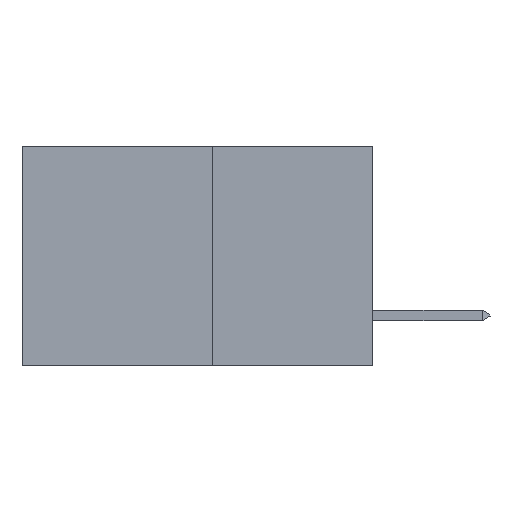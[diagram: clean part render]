
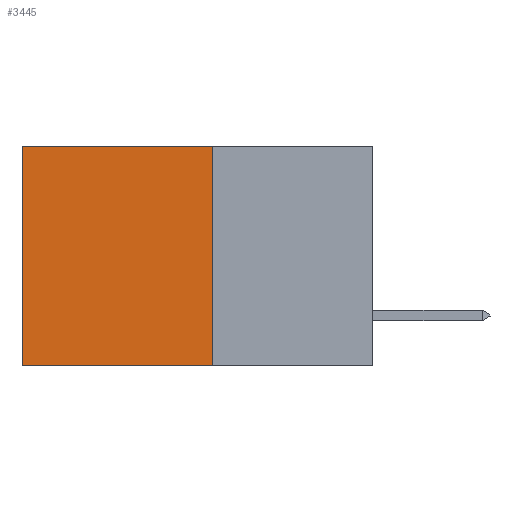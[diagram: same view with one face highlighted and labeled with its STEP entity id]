
A CAD part, left-side view. The second image highlights one B-rep face of the part: STEP entity #3445.
In plain terms, the highlighted planar face has unit normal (-1, 0, 0).
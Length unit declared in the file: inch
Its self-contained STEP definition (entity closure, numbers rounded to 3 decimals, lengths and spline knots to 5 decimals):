
#724 = ORIENTED_EDGE ( 'NONE', *, *, #5839, .F. ) ;
#1771 = VERTEX_POINT ( 'NONE', #5161 ) ;
#1816 = DIRECTION ( 'NONE',  ( 0., 0., -1. ) ) ;
#1899 = DIRECTION ( 'NONE',  ( 1., 0., 0. ) ) ;
#2190 = DIRECTION ( 'NONE',  ( 0., 1., 0. ) ) ;
#2387 = LINE ( 'NONE', #5983, #12265 ) ;
#2451 = PLANE ( 'NONE',  #14205 ) ;
#2814 = VECTOR ( 'NONE', #15606, 39.37008 ) ;
#2825 = CARTESIAN_POINT ( 'NONE',  ( 0.277, 0.27, -0.37 ) ) ;
#2922 = CARTESIAN_POINT ( 'NONE',  ( 0.277, 0.27, -0.37 ) ) ;
#3444 = EDGE_CURVE ( 'NONE', #1771, #4629, #15826, .T. ) ;
#3445 = ADVANCED_FACE ( 'NONE', ( #6402 ), #2451, .F. ) ;
#4629 = VERTEX_POINT ( 'NONE', #6544 ) ;
#5161 = CARTESIAN_POINT ( 'NONE',  ( 0.277, 0.27, -0.37 ) ) ;
#5839 = EDGE_CURVE ( 'NONE', #7050, #1771, #9433, .T. ) ;
#5983 = CARTESIAN_POINT ( 'NONE',  ( 0.277, 0.59, -0.37 ) ) ;
#6402 = FACE_OUTER_BOUND ( 'NONE', #15856, .T. ) ;
#6544 = CARTESIAN_POINT ( 'NONE',  ( 0.277, 0.59, -0.37 ) ) ;
#7050 = VERTEX_POINT ( 'NONE', #11337 ) ;
#7875 = VECTOR ( 'NONE', #11396, 39.37008 ) ;
#8386 = VERTEX_POINT ( 'NONE', #10908 ) ;
#9433 = LINE ( 'NONE', #15639, #2814 ) ;
#10185 = CARTESIAN_POINT ( 'NONE',  ( 0.277, 0.27, 0. ) ) ;
#10723 = ORIENTED_EDGE ( 'NONE', *, *, #13278, .T. ) ;
#10900 = DIRECTION ( 'NONE',  ( 0., 0., -1. ) ) ;
#10908 = CARTESIAN_POINT ( 'NONE',  ( 0.277, 0.59, 0. ) ) ;
#11141 = LINE ( 'NONE', #10185, #7875 ) ;
#11337 = CARTESIAN_POINT ( 'NONE',  ( 0.277, 0.27, 0. ) ) ;
#11396 = DIRECTION ( 'NONE',  ( 0., 1., 0. ) ) ;
#11452 = ORIENTED_EDGE ( 'NONE', *, *, #14411, .T. ) ;
#11821 = ORIENTED_EDGE ( 'NONE', *, *, #3444, .F. ) ;
#12265 = VECTOR ( 'NONE', #10900, 39.37008 ) ;
#12534 = VECTOR ( 'NONE', #2190, 39.37008 ) ;
#13278 = EDGE_CURVE ( 'NONE', #7050, #8386, #11141, .T. ) ;
#14205 = AXIS2_PLACEMENT_3D ( 'NONE', #2825, #1899, #1816 ) ;
#14411 = EDGE_CURVE ( 'NONE', #8386, #4629, #2387, .T. ) ;
#15606 = DIRECTION ( 'NONE',  ( 0., 0., -1. ) ) ;
#15639 = CARTESIAN_POINT ( 'NONE',  ( 0.277, 0.27, -0.37 ) ) ;
#15826 = LINE ( 'NONE', #2922, #12534 ) ;
#15856 = EDGE_LOOP ( 'NONE', ( #11452, #11821, #724, #10723 ) ) ;
